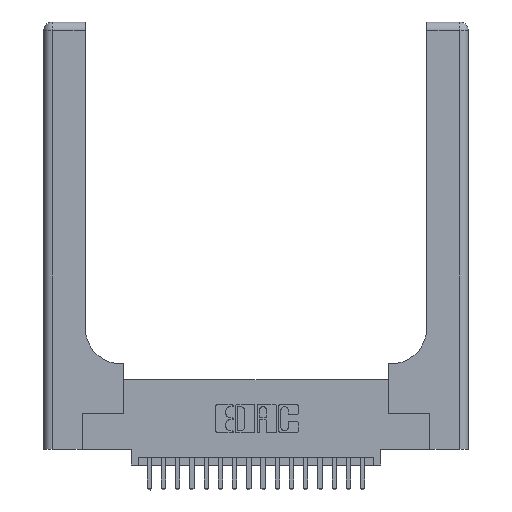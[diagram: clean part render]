
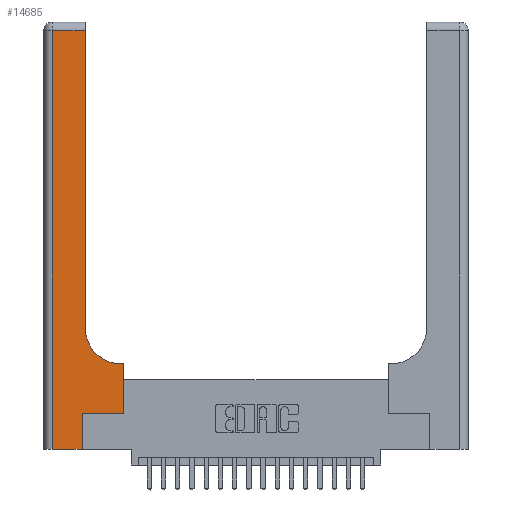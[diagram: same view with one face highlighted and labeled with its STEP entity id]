
A CAD part, top view. The second image highlights one B-rep face of the part: STEP entity #14685.
In plain terms, the highlighted planar face has unit normal (0, 0, 1).
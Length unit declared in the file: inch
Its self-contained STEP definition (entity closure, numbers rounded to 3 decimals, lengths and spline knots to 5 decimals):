
#300 = VECTOR ( 'NONE', #4069, 39.37008 ) ;
#657 = VERTEX_POINT ( 'NONE', #7422 ) ;
#660 = CARTESIAN_POINT ( 'NONE',  ( 0.2915, 2.94, 0.37 ) ) ;
#682 = CARTESIAN_POINT ( 'NONE',  ( 0., 0., 0.37 ) ) ;
#756 = DIRECTION ( 'NONE',  ( 0., 1., 0. ) ) ;
#792 = LINE ( 'NONE', #10695, #10658 ) ;
#903 = LINE ( 'NONE', #18135, #18030 ) ;
#1835 = AXIS2_PLACEMENT_3D ( 'NONE', #2593, #21100, #12817 ) ;
#2131 = VERTEX_POINT ( 'NONE', #11791 ) ;
#2238 = FACE_OUTER_BOUND ( 'NONE', #9986, .T. ) ;
#2498 = EDGE_CURVE ( 'NONE', #21496, #18483, #16512, .T. ) ;
#2593 = CARTESIAN_POINT ( 'NONE',  ( 0.5415, 0.85, 0.37 ) ) ;
#3118 = PLANE ( 'NONE',  #10017 ) ;
#3297 = DIRECTION ( 'NONE',  ( -1., 0., 0. ) ) ;
#3486 = ORIENTED_EDGE ( 'NONE', *, *, #10329, .T. ) ;
#4069 = DIRECTION ( 'NONE',  ( 1., 0., 0. ) ) ;
#4143 = EDGE_CURVE ( 'NONE', #5914, #657, #14970, .T. ) ;
#4157 = ORIENTED_EDGE ( 'NONE', *, *, #11774, .T. ) ;
#4235 = DIRECTION ( 'NONE',  ( 1., 0., 0. ) ) ;
#4237 = ORIENTED_EDGE ( 'NONE', *, *, #10235, .T. ) ;
#4625 = VERTEX_POINT ( 'NONE', #660 ) ;
#4852 = ORIENTED_EDGE ( 'NONE', *, *, #8281, .T. ) ;
#4973 = CARTESIAN_POINT ( 'NONE',  ( 0.2915, 0.6, 0.37 ) ) ;
#5914 = VERTEX_POINT ( 'NONE', #8781 ) ;
#6281 = ORIENTED_EDGE ( 'NONE', *, *, #4143, .T. ) ;
#6456 = CARTESIAN_POINT ( 'NONE',  ( 0.269, 0., 0.37 ) ) ;
#7057 = LINE ( 'NONE', #682, #300 ) ;
#7270 = ORIENTED_EDGE ( 'NONE', *, *, #18513, .T. ) ;
#7422 = CARTESIAN_POINT ( 'NONE',  ( 0.2915, 0.85, 0.37 ) ) ;
#7977 = DIRECTION ( 'NONE',  ( 0., 0., -1. ) ) ;
#8281 = EDGE_CURVE ( 'NONE', #18483, #15121, #7057, .T. ) ;
#8781 = CARTESIAN_POINT ( 'NONE',  ( 0.5415, 0.6, 0.37 ) ) ;
#8906 = CARTESIAN_POINT ( 'NONE',  ( 0.06, 3., 0.37 ) ) ;
#9157 = VECTOR ( 'NONE', #3297, 39.37008 ) ;
#9666 = CARTESIAN_POINT ( 'NONE',  ( 0.269, 0., 0.37 ) ) ;
#9774 = DIRECTION ( 'NONE',  ( 0., 1., 0. ) ) ;
#9784 = ORIENTED_EDGE ( 'NONE', *, *, #15669, .T. ) ;
#9950 = CARTESIAN_POINT ( 'NONE',  ( 0.5585, 0.25, 0.37 ) ) ;
#9986 = EDGE_LOOP ( 'NONE', ( #3486, #16034, #16431, #4852, #7270, #4157, #9784, #4237, #6281 ) ) ;
#10012 = LINE ( 'NONE', #18963, #18335 ) ;
#10017 = AXIS2_PLACEMENT_3D ( 'NONE', #14706, #7977, #19803 ) ;
#10225 = CARTESIAN_POINT ( 'NONE',  ( 0.5585, 0.6, 0.37 ) ) ;
#10235 = EDGE_CURVE ( 'NONE', #10424, #5914, #10739, .T. ) ;
#10329 = EDGE_CURVE ( 'NONE', #657, #4625, #19838, .T. ) ;
#10424 = VERTEX_POINT ( 'NONE', #10225 ) ;
#10658 = VECTOR ( 'NONE', #4235, 39.37008 ) ;
#10695 = CARTESIAN_POINT ( 'NONE',  ( 0.269, 0.25, 0.37 ) ) ;
#10739 = LINE ( 'NONE', #4973, #9157 ) ;
#11566 = VECTOR ( 'NONE', #14896, 39.37008 ) ;
#11774 = EDGE_CURVE ( 'NONE', #2131, #13530, #792, .T. ) ;
#11791 = CARTESIAN_POINT ( 'NONE',  ( 0.269, 0.25, 0.37 ) ) ;
#12817 = DIRECTION ( 'NONE',  ( 1., 0., 0. ) ) ;
#13031 = CARTESIAN_POINT ( 'NONE',  ( 0.06, 2.94, 0.37 ) ) ;
#13286 = DIRECTION ( 'NONE',  ( 0., 1., 0. ) ) ;
#13351 = CARTESIAN_POINT ( 'NONE',  ( 0.2915, 3., 0.37 ) ) ;
#13530 = VERTEX_POINT ( 'NONE', #9950 ) ;
#13817 = VECTOR ( 'NONE', #13286, 39.37008 ) ;
#14685 = ADVANCED_FACE ( 'NONE', ( #2238 ), #3118, .F. ) ;
#14706 = CARTESIAN_POINT ( 'NONE',  ( 0., 3., 0.37 ) ) ;
#14896 = DIRECTION ( 'NONE',  ( 0., -1., 0. ) ) ;
#14970 = CIRCLE ( 'NONE', #1835, 0.25 ) ;
#15121 = VERTEX_POINT ( 'NONE', #9666 ) ;
#15669 = EDGE_CURVE ( 'NONE', #13530, #10424, #10012, .T. ) ;
#16034 = ORIENTED_EDGE ( 'NONE', *, *, #16385, .T. ) ;
#16385 = EDGE_CURVE ( 'NONE', #4625, #21496, #903, .T. ) ;
#16431 = ORIENTED_EDGE ( 'NONE', *, *, #2498, .T. ) ;
#16512 = LINE ( 'NONE', #8906, #11566 ) ;
#17922 = CARTESIAN_POINT ( 'NONE',  ( 0.06, 0., 0.37 ) ) ;
#18030 = VECTOR ( 'NONE', #21485, 39.37008 ) ;
#18135 = CARTESIAN_POINT ( 'NONE',  ( 0., 2.94, 0.37 ) ) ;
#18335 = VECTOR ( 'NONE', #756, 39.37008 ) ;
#18483 = VERTEX_POINT ( 'NONE', #17922 ) ;
#18513 = EDGE_CURVE ( 'NONE', #15121, #2131, #21202, .T. ) ;
#18963 = CARTESIAN_POINT ( 'NONE',  ( 0.5585, 0.25, 0.37 ) ) ;
#19803 = DIRECTION ( 'NONE',  ( -1., 0., 0. ) ) ;
#19838 = LINE ( 'NONE', #13351, #13817 ) ;
#20963 = VECTOR ( 'NONE', #9774, 39.37008 ) ;
#21100 = DIRECTION ( 'NONE',  ( 0., 0., -1. ) ) ;
#21202 = LINE ( 'NONE', #6456, #20963 ) ;
#21485 = DIRECTION ( 'NONE',  ( -1., 0., 0. ) ) ;
#21496 = VERTEX_POINT ( 'NONE', #13031 ) ;
